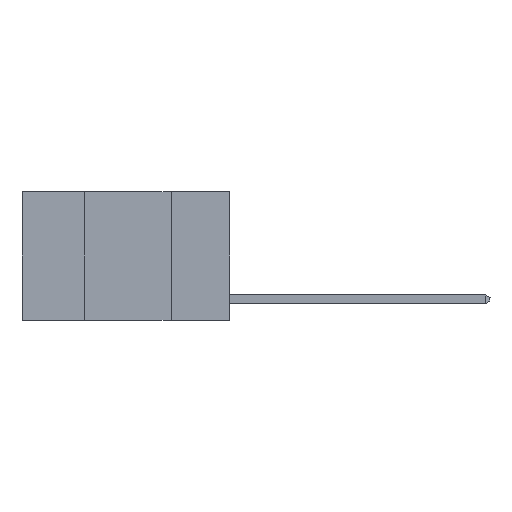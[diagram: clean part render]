
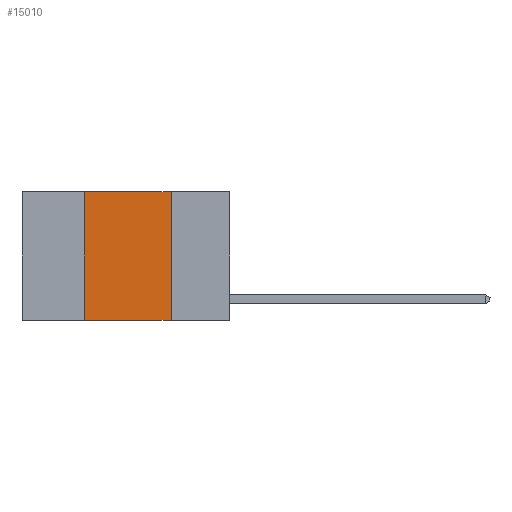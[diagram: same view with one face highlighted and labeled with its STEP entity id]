
A CAD part, left-side view. The second image highlights one B-rep face of the part: STEP entity #15010.
In plain terms, the highlighted planar face has unit normal (-1, 0, 0).
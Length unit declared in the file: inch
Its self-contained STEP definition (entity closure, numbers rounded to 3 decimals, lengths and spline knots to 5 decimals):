
#124 = DIRECTION ( 'NONE',  ( 0., 0., 1. ) ) ;
#172 = CARTESIAN_POINT ( 'NONE',  ( 0., 0.17, -0.37 ) ) ;
#1009 = VERTEX_POINT ( 'NONE', #11639 ) ;
#1680 = VECTOR ( 'NONE', #7753, 39.37008 ) ;
#2157 = VERTEX_POINT ( 'NONE', #172 ) ;
#2422 = CARTESIAN_POINT ( 'NONE',  ( 0., 0.17, 0. ) ) ;
#2797 = CARTESIAN_POINT ( 'NONE',  ( 0., 0.17, 0. ) ) ;
#3251 = PLANE ( 'NONE',  #8242 ) ;
#4284 = EDGE_CURVE ( 'NONE', #1009, #2157, #10658, .T. ) ;
#5252 = VERTEX_POINT ( 'NONE', #2797 ) ;
#5364 = LINE ( 'NONE', #2422, #14443 ) ;
#5381 = VERTEX_POINT ( 'NONE', #14514 ) ;
#5651 = DIRECTION ( 'NONE',  ( 0., 0., -1. ) ) ;
#6373 = ORIENTED_EDGE ( 'NONE', *, *, #13517, .F. ) ;
#6595 = CARTESIAN_POINT ( 'NONE',  ( 0., 0.6, -0.37 ) ) ;
#6984 = VECTOR ( 'NONE', #12141, 39.37008 ) ;
#7753 = DIRECTION ( 'NONE',  ( 0., -1., 0. ) ) ;
#8207 = FACE_OUTER_BOUND ( 'NONE', #13834, .T. ) ;
#8242 = AXIS2_PLACEMENT_3D ( 'NONE', #11360, #12491, #5651 ) ;
#8466 = CARTESIAN_POINT ( 'NONE',  ( 0., 0.42, 0. ) ) ;
#9789 = ORIENTED_EDGE ( 'NONE', *, *, #11259, .F. ) ;
#10042 = LINE ( 'NONE', #10996, #6984 ) ;
#10049 = EDGE_CURVE ( 'NONE', #5381, #5252, #10042, .T. ) ;
#10597 = DIRECTION ( 'NONE',  ( 0., 0., -1. ) ) ;
#10658 = LINE ( 'NONE', #6595, #1680 ) ;
#10996 = CARTESIAN_POINT ( 'NONE',  ( 0., 0.6, 0. ) ) ;
#11259 = EDGE_CURVE ( 'NONE', #1009, #5381, #11356, .T. ) ;
#11356 = LINE ( 'NONE', #8466, #13626 ) ;
#11360 = CARTESIAN_POINT ( 'NONE',  ( 0., 0.6, 0. ) ) ;
#11639 = CARTESIAN_POINT ( 'NONE',  ( 0., 0.42, -0.37 ) ) ;
#12141 = DIRECTION ( 'NONE',  ( 0., -1., 0. ) ) ;
#12429 = ORIENTED_EDGE ( 'NONE', *, *, #10049, .F. ) ;
#12491 = DIRECTION ( 'NONE',  ( 1., 0., 0. ) ) ;
#12788 = ORIENTED_EDGE ( 'NONE', *, *, #4284, .T. ) ;
#13517 = EDGE_CURVE ( 'NONE', #5252, #2157, #5364, .T. ) ;
#13626 = VECTOR ( 'NONE', #124, 39.37008 ) ;
#13834 = EDGE_LOOP ( 'NONE', ( #6373, #12429, #9789, #12788 ) ) ;
#14443 = VECTOR ( 'NONE', #10597, 39.37008 ) ;
#14514 = CARTESIAN_POINT ( 'NONE',  ( 0., 0.42, 0. ) ) ;
#15010 = ADVANCED_FACE ( 'NONE', ( #8207 ), #3251, .F. ) ;
